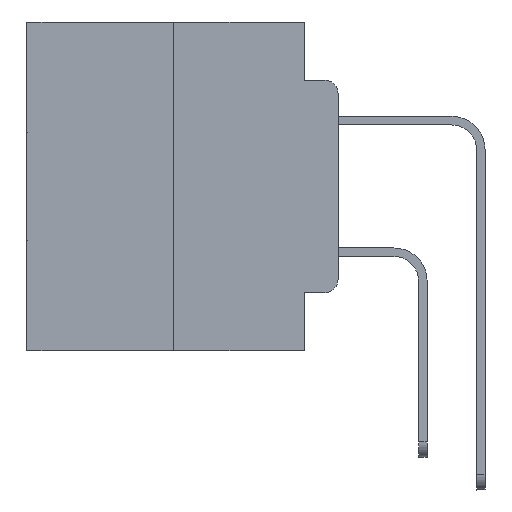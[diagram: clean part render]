
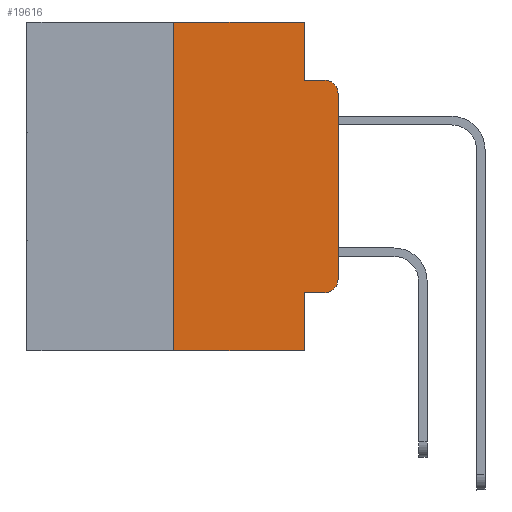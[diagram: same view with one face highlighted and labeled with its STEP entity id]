
A CAD part, left-side view. The second image highlights one B-rep face of the part: STEP entity #19616.
In plain terms, the highlighted planar face has unit normal (-1, 0, 0).
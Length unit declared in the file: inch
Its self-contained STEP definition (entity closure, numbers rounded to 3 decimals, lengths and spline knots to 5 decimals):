
#97 = LINE ( 'NONE', #23303, #5763 ) ;
#702 = CARTESIAN_POINT ( 'NONE',  ( 0., 0.051, -0.5 ) ) ;
#890 = ORIENTED_EDGE ( 'NONE', *, *, #11343, .T. ) ;
#1256 = CARTESIAN_POINT ( 'NONE',  ( 0., 0., 0. ) ) ;
#2254 = DIRECTION ( 'NONE',  ( 0., 0., -1. ) ) ;
#2667 = CARTESIAN_POINT ( 'NONE',  ( 0., 0.02, -0.3915 ) ) ;
#2712 = CARTESIAN_POINT ( 'NONE',  ( 0., 0., -0.1085 ) ) ;
#3185 = CARTESIAN_POINT ( 'NONE',  ( 0., 0.051, -0.4115 ) ) ;
#3223 = ORIENTED_EDGE ( 'NONE', *, *, #8107, .T. ) ;
#3397 = EDGE_CURVE ( 'NONE', #15733, #7502, #10087, .T. ) ;
#3790 = VECTOR ( 'NONE', #15761, 39.37008 ) ;
#3886 = CARTESIAN_POINT ( 'NONE',  ( 0., 0.051, 0. ) ) ;
#4499 = VERTEX_POINT ( 'NONE', #3185 ) ;
#4579 = PLANE ( 'NONE',  #7979 ) ;
#5052 = DIRECTION ( 'NONE',  ( 0., 0., -1. ) ) ;
#5071 = ORIENTED_EDGE ( 'NONE', *, *, #13715, .F. ) ;
#5763 = VECTOR ( 'NONE', #14025, 39.37008 ) ;
#5960 = CARTESIAN_POINT ( 'NONE',  ( 0., 0., -0.3915 ) ) ;
#6270 = LINE ( 'NONE', #19511, #11848 ) ;
#6296 = VECTOR ( 'NONE', #24837, 39.37008 ) ;
#6556 = EDGE_CURVE ( 'NONE', #7502, #9756, #97, .T. ) ;
#6799 = LINE ( 'NONE', #19592, #24035 ) ;
#7502 = VERTEX_POINT ( 'NONE', #17460 ) ;
#7580 = EDGE_LOOP ( 'NONE', ( #890, #3223, #17255, #27757, #5071, #8787, #21291, #17285, #30231, #27070 ) ) ;
#7769 = DIRECTION ( 'NONE',  ( 0., 0., 1. ) ) ;
#7976 = VECTOR ( 'NONE', #15614, 39.37008 ) ;
#7979 = AXIS2_PLACEMENT_3D ( 'NONE', #30237, #16468, #2254 ) ;
#8107 = EDGE_CURVE ( 'NONE', #24410, #9756, #29374, .T. ) ;
#8787 = ORIENTED_EDGE ( 'NONE', *, *, #29008, .F. ) ;
#9756 = VERTEX_POINT ( 'NONE', #16513 ) ;
#10087 = LINE ( 'NONE', #13374, #3790 ) ;
#10865 = CARTESIAN_POINT ( 'NONE',  ( 0., 0.02, -0.1085 ) ) ;
#11343 = EDGE_CURVE ( 'NONE', #26980, #24410, #12593, .T. ) ;
#11848 = VECTOR ( 'NONE', #7769, 39.37008 ) ;
#12593 = LINE ( 'NONE', #1256, #6296 ) ;
#13073 = VERTEX_POINT ( 'NONE', #24980 ) ;
#13216 = DIRECTION ( 'NONE',  ( 0., 0., -1. ) ) ;
#13237 = CARTESIAN_POINT ( 'NONE',  ( 0., 0.473, 0. ) ) ;
#13374 = CARTESIAN_POINT ( 'NONE',  ( 0., 0.051, 0. ) ) ;
#13715 = EDGE_CURVE ( 'NONE', #26108, #15733, #15042, .T. ) ;
#14025 = DIRECTION ( 'NONE',  ( 0., -1., 0. ) ) ;
#15042 = LINE ( 'NONE', #13237, #7976 ) ;
#15614 = DIRECTION ( 'NONE',  ( 0., -1., 0. ) ) ;
#15733 = VERTEX_POINT ( 'NONE', #23865 ) ;
#15761 = DIRECTION ( 'NONE',  ( 0., 0., -1. ) ) ;
#16272 = CARTESIAN_POINT ( 'NONE',  ( 0., 0.25, 0. ) ) ;
#16468 = DIRECTION ( 'NONE',  ( 1., 0., 0. ) ) ;
#16513 = CARTESIAN_POINT ( 'NONE',  ( 0., 0.02, -0.0885 ) ) ;
#16971 = CARTESIAN_POINT ( 'NONE',  ( 0., 0.051, -0.4115 ) ) ;
#17255 = ORIENTED_EDGE ( 'NONE', *, *, #6556, .F. ) ;
#17285 = ORIENTED_EDGE ( 'NONE', *, *, #25973, .F. ) ;
#17460 = CARTESIAN_POINT ( 'NONE',  ( 0., 0.051, -0.0885 ) ) ;
#17472 = AXIS2_PLACEMENT_3D ( 'NONE', #10865, #27133, #13216 ) ;
#17675 = CARTESIAN_POINT ( 'NONE',  ( 0., 0.02, -0.4115 ) ) ;
#19176 = DIRECTION ( 'NONE',  ( -1., 0., 0. ) ) ;
#19307 = DIRECTION ( 'NONE',  ( 0., -1., 0. ) ) ;
#19511 = CARTESIAN_POINT ( 'NONE',  ( 0., 0.25, 0. ) ) ;
#19592 = CARTESIAN_POINT ( 'NONE',  ( 0., 0.473, -0.5 ) ) ;
#19616 = ADVANCED_FACE ( 'NONE', ( #21735 ), #4579, .F. ) ;
#20459 = DIRECTION ( 'NONE',  ( 0., 0., -1. ) ) ;
#21291 = ORIENTED_EDGE ( 'NONE', *, *, #26366, .T. ) ;
#21735 = FACE_OUTER_BOUND ( 'NONE', #7580, .T. ) ;
#21943 = DIRECTION ( 'NONE',  ( 0., -1., 0. ) ) ;
#22496 = VERTEX_POINT ( 'NONE', #17675 ) ;
#22873 = EDGE_CURVE ( 'NONE', #22496, #26980, #28907, .T. ) ;
#23022 = VERTEX_POINT ( 'NONE', #702 ) ;
#23092 = VECTOR ( 'NONE', #19307, 39.37008 ) ;
#23303 = CARTESIAN_POINT ( 'NONE',  ( 0., 0.051, -0.0885 ) ) ;
#23352 = VECTOR ( 'NONE', #20459, 39.37008 ) ;
#23865 = CARTESIAN_POINT ( 'NONE',  ( 0., 0.051, 0. ) ) ;
#24035 = VECTOR ( 'NONE', #21943, 39.37008 ) ;
#24062 = LINE ( 'NONE', #3886, #23352 ) ;
#24410 = VERTEX_POINT ( 'NONE', #2712 ) ;
#24418 = EDGE_CURVE ( 'NONE', #4499, #22496, #29879, .T. ) ;
#24837 = DIRECTION ( 'NONE',  ( 0., 0., 1. ) ) ;
#24980 = CARTESIAN_POINT ( 'NONE',  ( 0., 0.25, -0.5 ) ) ;
#25703 = AXIS2_PLACEMENT_3D ( 'NONE', #2667, #19176, #5052 ) ;
#25973 = EDGE_CURVE ( 'NONE', #4499, #23022, #24062, .T. ) ;
#26108 = VERTEX_POINT ( 'NONE', #16272 ) ;
#26366 = EDGE_CURVE ( 'NONE', #13073, #23022, #6799, .T. ) ;
#26980 = VERTEX_POINT ( 'NONE', #5960 ) ;
#27070 = ORIENTED_EDGE ( 'NONE', *, *, #22873, .T. ) ;
#27133 = DIRECTION ( 'NONE',  ( -1., 0., 0. ) ) ;
#27757 = ORIENTED_EDGE ( 'NONE', *, *, #3397, .F. ) ;
#28907 = CIRCLE ( 'NONE', #25703, 0.02 ) ;
#29008 = EDGE_CURVE ( 'NONE', #13073, #26108, #6270, .T. ) ;
#29374 = CIRCLE ( 'NONE', #17472, 0.02 ) ;
#29879 = LINE ( 'NONE', #16971, #23092 ) ;
#30231 = ORIENTED_EDGE ( 'NONE', *, *, #24418, .T. ) ;
#30237 = CARTESIAN_POINT ( 'NONE',  ( 0., 0.473, 0. ) ) ;
